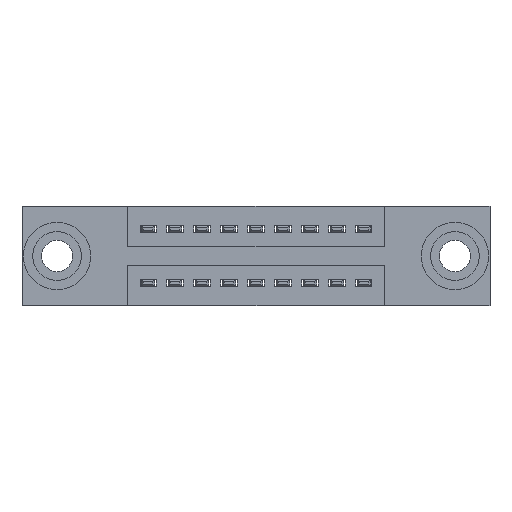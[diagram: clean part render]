
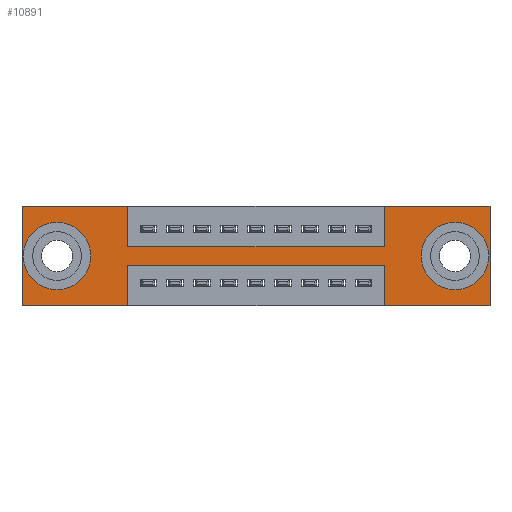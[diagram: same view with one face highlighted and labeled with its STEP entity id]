
A CAD part, front view. The second image highlights one B-rep face of the part: STEP entity #10891.
In plain terms, the highlighted planar face has unit normal (0, -1, 0).
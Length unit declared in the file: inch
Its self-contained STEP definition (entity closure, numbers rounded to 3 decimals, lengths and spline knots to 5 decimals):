
#16 = CIRCLE ( 'NONE', #9846, 0.078 ) ;
#35 = EDGE_CURVE ( 'NONE', #6112, #667, #7105, .T. ) ;
#111 = DIRECTION ( 'NONE',  ( 0., 0., -1. ) ) ;
#116 = DIRECTION ( 'NONE',  ( 0., 0., -1. ) ) ;
#165 = DIRECTION ( 'NONE',  ( 0., 0., 1. ) ) ;
#168 = EDGE_CURVE ( 'NONE', #6444, #6378, #16, .T. ) ;
#204 = DIRECTION ( 'NONE',  ( 0., 1., 0. ) ) ;
#381 = FACE_BOUND ( 'NONE', #11183, .T. ) ;
#495 = CARTESIAN_POINT ( 'NONE',  ( 1.735, 0., 0. ) ) ;
#507 = VECTOR ( 'NONE', #3628, 39.37008 ) ;
#625 = CARTESIAN_POINT ( 'NONE',  ( 1.605, 0., -0.263 ) ) ;
#667 = VERTEX_POINT ( 'NONE', #1736 ) ;
#848 = ORIENTED_EDGE ( 'NONE', *, *, #168, .T. ) ;
#943 = EDGE_LOOP ( 'NONE', ( #2020, #8210 ) ) ;
#1003 = DIRECTION ( 'NONE',  ( 0., 1., 0. ) ) ;
#1023 = CARTESIAN_POINT ( 'NONE',  ( 0.13, 0., -0.185 ) ) ;
#1051 = CARTESIAN_POINT ( 'NONE',  ( 0.3925, 0., -0.15 ) ) ;
#1111 = ORIENTED_EDGE ( 'NONE', *, *, #10348, .F. ) ;
#1445 = CIRCLE ( 'NONE', #11625, 0.078 ) ;
#1736 = CARTESIAN_POINT ( 'NONE',  ( 0., 0., 0. ) ) ;
#1745 = CARTESIAN_POINT ( 'NONE',  ( 1.3425, 0., -0.15 ) ) ;
#1791 = CARTESIAN_POINT ( 'NONE',  ( 0., 0., 0. ) ) ;
#1807 = VERTEX_POINT ( 'NONE', #10060 ) ;
#1820 = VECTOR ( 'NONE', #6269, 39.37008 ) ;
#1987 = CIRCLE ( 'NONE', #3049, 0.078 ) ;
#2020 = ORIENTED_EDGE ( 'NONE', *, *, #5779, .T. ) ;
#2125 = CARTESIAN_POINT ( 'NONE',  ( 0., 0., -0.37 ) ) ;
#2133 = LINE ( 'NONE', #495, #11713 ) ;
#2224 = DIRECTION ( 'NONE',  ( 0., -1., 0. ) ) ;
#2245 = ORIENTED_EDGE ( 'NONE', *, *, #6214, .F. ) ;
#2257 = CARTESIAN_POINT ( 'NONE',  ( 1.3425, 0., 0. ) ) ;
#2515 = DIRECTION ( 'NONE',  ( 1., 0., 0. ) ) ;
#2522 = CARTESIAN_POINT ( 'NONE',  ( 1.735, 0., -0.37 ) ) ;
#2983 = FACE_BOUND ( 'NONE', #943, .T. ) ;
#3049 = AXIS2_PLACEMENT_3D ( 'NONE', #3240, #1003, #4209 ) ;
#3134 = CARTESIAN_POINT ( 'NONE',  ( 0., 0., -0.37 ) ) ;
#3186 = EDGE_CURVE ( 'NONE', #7154, #4571, #7335, .T. ) ;
#3226 = DIRECTION ( 'NONE',  ( -1., 0., 0. ) ) ;
#3240 = CARTESIAN_POINT ( 'NONE',  ( 1.605, 0., -0.185 ) ) ;
#3438 = CARTESIAN_POINT ( 'NONE',  ( 1.3425, 0., 0. ) ) ;
#3612 = CARTESIAN_POINT ( 'NONE',  ( 1.3425, 0., -0.37 ) ) ;
#3628 = DIRECTION ( 'NONE',  ( -1., 0., 0. ) ) ;
#3672 = EDGE_CURVE ( 'NONE', #8976, #11906, #10001, .T. ) ;
#3712 = CARTESIAN_POINT ( 'NONE',  ( 0., 0., -0.37 ) ) ;
#3732 = ORIENTED_EDGE ( 'NONE', *, *, #6366, .F. ) ;
#3816 = CIRCLE ( 'NONE', #4056, 0.078 ) ;
#3863 = ORIENTED_EDGE ( 'NONE', *, *, #11591, .F. ) ;
#3920 = CARTESIAN_POINT ( 'NONE',  ( 1.3425, 0., -0.37 ) ) ;
#4056 = AXIS2_PLACEMENT_3D ( 'NONE', #1023, #7620, #165 ) ;
#4108 = LINE ( 'NONE', #10317, #9675 ) ;
#4124 = VERTEX_POINT ( 'NONE', #10855 ) ;
#4209 = DIRECTION ( 'NONE',  ( 0., 0., -1. ) ) ;
#4427 = DIRECTION ( 'NONE',  ( 0., 0., 1. ) ) ;
#4488 = EDGE_CURVE ( 'NONE', #11906, #6943, #2133, .T. ) ;
#4550 = VECTOR ( 'NONE', #3226, 39.37008 ) ;
#4571 = VERTEX_POINT ( 'NONE', #8082 ) ;
#4722 = DIRECTION ( 'NONE',  ( 1., 0., 0. ) ) ;
#4728 = DIRECTION ( 'NONE',  ( 0., 1., 0. ) ) ;
#4741 = CARTESIAN_POINT ( 'NONE',  ( 0.3925, 0., -0.15 ) ) ;
#4845 = CARTESIAN_POINT ( 'NONE',  ( 0.13, 0., -0.185 ) ) ;
#4891 = VECTOR ( 'NONE', #2515, 39.37008 ) ;
#5110 = FACE_OUTER_BOUND ( 'NONE', #7134, .T. ) ;
#5276 = EDGE_CURVE ( 'NONE', #7017, #10327, #8235, .T. ) ;
#5570 = DIRECTION ( 'NONE',  ( 0., 0., 1. ) ) ;
#5678 = LINE ( 'NONE', #3438, #8314 ) ;
#5733 = VERTEX_POINT ( 'NONE', #625 ) ;
#5734 = CARTESIAN_POINT ( 'NONE',  ( 1.605, 0., -0.185 ) ) ;
#5740 = VECTOR ( 'NONE', #116, 39.37008 ) ;
#5779 = EDGE_CURVE ( 'NONE', #4124, #5733, #1987, .T. ) ;
#5786 = PLANE ( 'NONE',  #10770 ) ;
#5860 = VECTOR ( 'NONE', #4722, 39.37008 ) ;
#5895 = CARTESIAN_POINT ( 'NONE',  ( 0., 0., -0.37 ) ) ;
#5976 = VERTEX_POINT ( 'NONE', #1745 ) ;
#6112 = VERTEX_POINT ( 'NONE', #2125 ) ;
#6214 = EDGE_CURVE ( 'NONE', #4571, #9992, #4108, .T. ) ;
#6269 = DIRECTION ( 'NONE',  ( 0., 0., 1. ) ) ;
#6366 = EDGE_CURVE ( 'NONE', #667, #7017, #8071, .T. ) ;
#6378 = VERTEX_POINT ( 'NONE', #6568 ) ;
#6444 = VERTEX_POINT ( 'NONE', #11218 ) ;
#6540 = EDGE_CURVE ( 'NONE', #1807, #6112, #7634, .T. ) ;
#6568 = CARTESIAN_POINT ( 'NONE',  ( 0.13, 0., -0.263 ) ) ;
#6644 = DIRECTION ( 'NONE',  ( 0., 0., -1. ) ) ;
#6943 = VERTEX_POINT ( 'NONE', #2522 ) ;
#6964 = LINE ( 'NONE', #11325, #9174 ) ;
#7017 = VERTEX_POINT ( 'NONE', #9239 ) ;
#7105 = LINE ( 'NONE', #1791, #8166 ) ;
#7134 = EDGE_LOOP ( 'NONE', ( #11536, #2245, #11640, #3863, #10982, #9537, #7908, #1111, #11186, #3732, #9296, #7774 ) ) ;
#7154 = VERTEX_POINT ( 'NONE', #3920 ) ;
#7191 = CARTESIAN_POINT ( 'NONE',  ( 0., 0., 0. ) ) ;
#7335 = LINE ( 'NONE', #3612, #1820 ) ;
#7620 = DIRECTION ( 'NONE',  ( 0., 1., 0. ) ) ;
#7634 = LINE ( 'NONE', #5895, #4550 ) ;
#7774 = ORIENTED_EDGE ( 'NONE', *, *, #6540, .F. ) ;
#7908 = ORIENTED_EDGE ( 'NONE', *, *, #8204, .F. ) ;
#8071 = LINE ( 'NONE', #11342, #5860 ) ;
#8082 = CARTESIAN_POINT ( 'NONE',  ( 1.3425, 0., -0.22 ) ) ;
#8166 = VECTOR ( 'NONE', #9714, 39.37008 ) ;
#8204 = EDGE_CURVE ( 'NONE', #5976, #8976, #5678, .T. ) ;
#8210 = ORIENTED_EDGE ( 'NONE', *, *, #9775, .T. ) ;
#8235 = LINE ( 'NONE', #9317, #5740 ) ;
#8314 = VECTOR ( 'NONE', #4427, 39.37008 ) ;
#8342 = DIRECTION ( 'NONE',  ( 1., 0., 0. ) ) ;
#8398 = EDGE_CURVE ( 'NONE', #9992, #1807, #6964, .T. ) ;
#8947 = CARTESIAN_POINT ( 'NONE',  ( 1.735, 0., 0. ) ) ;
#8976 = VERTEX_POINT ( 'NONE', #2257 ) ;
#9174 = VECTOR ( 'NONE', #111, 39.37008 ) ;
#9239 = CARTESIAN_POINT ( 'NONE',  ( 0.3925, 0., 0. ) ) ;
#9296 = ORIENTED_EDGE ( 'NONE', *, *, #35, .F. ) ;
#9317 = CARTESIAN_POINT ( 'NONE',  ( 0.3925, 0., 0. ) ) ;
#9537 = ORIENTED_EDGE ( 'NONE', *, *, #3672, .F. ) ;
#9659 = DIRECTION ( 'NONE',  ( 0., 0., -1. ) ) ;
#9675 = VECTOR ( 'NONE', #10235, 39.37008 ) ;
#9714 = DIRECTION ( 'NONE',  ( 0., 0., 1. ) ) ;
#9775 = EDGE_CURVE ( 'NONE', #5733, #4124, #1445, .T. ) ;
#9846 = AXIS2_PLACEMENT_3D ( 'NONE', #4845, #4728, #5570 ) ;
#9947 = VECTOR ( 'NONE', #8342, 39.37008 ) ;
#9992 = VERTEX_POINT ( 'NONE', #11813 ) ;
#10001 = LINE ( 'NONE', #7191, #4891 ) ;
#10060 = CARTESIAN_POINT ( 'NONE',  ( 0.3925, 0., -0.37 ) ) ;
#10235 = DIRECTION ( 'NONE',  ( -1., 0., 0. ) ) ;
#10317 = CARTESIAN_POINT ( 'NONE',  ( 0.3925, 0., -0.22 ) ) ;
#10327 = VERTEX_POINT ( 'NONE', #1051 ) ;
#10348 = EDGE_CURVE ( 'NONE', #10327, #5976, #10806, .T. ) ;
#10476 = EDGE_CURVE ( 'NONE', #6378, #6444, #3816, .T. ) ;
#10635 = DIRECTION ( 'NONE',  ( 0., 0., -1. ) ) ;
#10770 = AXIS2_PLACEMENT_3D ( 'NONE', #3134, #2224, #10635 ) ;
#10806 = LINE ( 'NONE', #4741, #9947 ) ;
#10855 = CARTESIAN_POINT ( 'NONE',  ( 1.605, 0., -0.107 ) ) ;
#10891 = ADVANCED_FACE ( 'NONE', ( #2983, #381, #5110 ), #5786, .T. ) ;
#10982 = ORIENTED_EDGE ( 'NONE', *, *, #4488, .F. ) ;
#11183 = EDGE_LOOP ( 'NONE', ( #848, #11699 ) ) ;
#11186 = ORIENTED_EDGE ( 'NONE', *, *, #5276, .F. ) ;
#11218 = CARTESIAN_POINT ( 'NONE',  ( 0.13, 0., -0.107 ) ) ;
#11325 = CARTESIAN_POINT ( 'NONE',  ( 0.3925, 0., -0.37 ) ) ;
#11342 = CARTESIAN_POINT ( 'NONE',  ( 0., 0., 0. ) ) ;
#11536 = ORIENTED_EDGE ( 'NONE', *, *, #8398, .F. ) ;
#11591 = EDGE_CURVE ( 'NONE', #6943, #7154, #11665, .T. ) ;
#11625 = AXIS2_PLACEMENT_3D ( 'NONE', #5734, #204, #6644 ) ;
#11640 = ORIENTED_EDGE ( 'NONE', *, *, #3186, .F. ) ;
#11665 = LINE ( 'NONE', #3712, #507 ) ;
#11699 = ORIENTED_EDGE ( 'NONE', *, *, #10476, .T. ) ;
#11713 = VECTOR ( 'NONE', #9659, 39.37008 ) ;
#11813 = CARTESIAN_POINT ( 'NONE',  ( 0.3925, 0., -0.22 ) ) ;
#11906 = VERTEX_POINT ( 'NONE', #8947 ) ;
